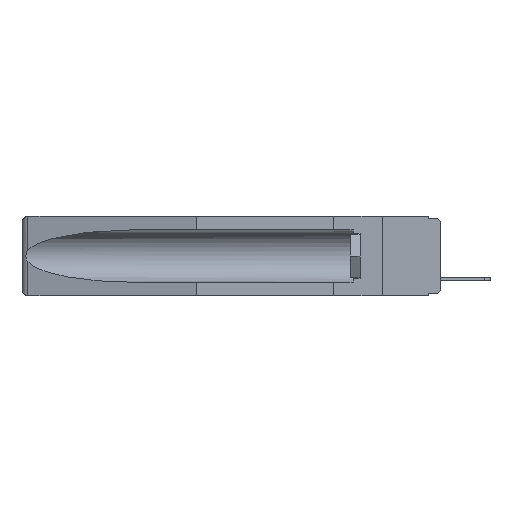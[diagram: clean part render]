
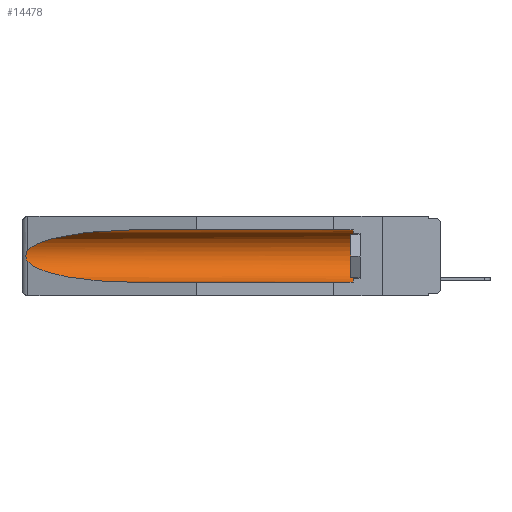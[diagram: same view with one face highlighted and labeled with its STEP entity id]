
A CAD part, left-side view. The second image highlights one B-rep face of the part: STEP entity #14478.
In plain terms, the highlighted cylindrical face has radius 2.857 mm (diameter 5.715 mm), a partial arc.
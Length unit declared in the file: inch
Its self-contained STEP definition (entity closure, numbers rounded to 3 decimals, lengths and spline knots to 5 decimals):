
#69 = CARTESIAN_POINT ( 'NONE',  ( 0.21114, 1.30732, -0.284 ) ) ;
#1136 = CARTESIAN_POINT ( 'NONE',  ( 0.2675, 1.53308, -0.17534 ) ) ;
#1635 = CIRCLE ( 'NONE', #4038, 0.1125 ) ;
#2344 = ORIENTED_EDGE ( 'NONE', *, *, #16342, .T. ) ;
#2562 = CARTESIAN_POINT ( 'NONE',  ( 0.2673, 1.5327, -0.16383 ) ) ;
#2883 = VERTEX_POINT ( 'NONE', #8727 ) ;
#2913 = CARTESIAN_POINT ( 'NONE',  ( 0.155, 1.07973, -0.059 ) ) ;
#2951 = VERTEX_POINT ( 'NONE', #15266 ) ;
#3969 = CARTESIAN_POINT ( 'NONE',  ( 0.26537, 1.52718, -0.14972 ) ) ;
#4036 = DIRECTION ( 'NONE',  ( 0., 1., 0. ) ) ;
#4038 = AXIS2_PLACEMENT_3D ( 'NONE', #18597, #11522, #12834 ) ;
#4839 = EDGE_CURVE ( 'NONE', #2883, #8540, #10561, .T. ) ;
#5042 = CARTESIAN_POINT ( 'NONE',  ( 0.155, -0.30754, -0.1715 ) ) ;
#5213 = VERTEX_POINT ( 'NONE', #5336 ) ;
#5292 = CARTESIAN_POINT ( 'NONE',  ( 0.155, 1.07973, -0.284 ) ) ;
#5336 = CARTESIAN_POINT ( 'NONE',  ( 0.155, 0.126, -0.059 ) ) ;
#5337 = ORIENTED_EDGE ( 'NONE', *, *, #6023, .T. ) ;
#5570 = CARTESIAN_POINT ( 'NONE',  ( 0.26537, 1.52718, -0.19328 ) ) ;
#6023 = EDGE_CURVE ( 'NONE', #2951, #2883, #7710, .T. ) ;
#6224 = CARTESIAN_POINT ( 'NONE',  ( 0.26537, 1.52718, -0.14972 ) ) ;
#6354 = CYLINDRICAL_SURFACE ( 'NONE', #13358, 0.1125 ) ;
#6381 = LINE ( 'NONE', #10812, #17502 ) ;
#6879 = CARTESIAN_POINT ( 'NONE',  ( 0.2673, 1.53269, -0.17917 ) ) ;
#6930 = VECTOR ( 'NONE', #17506, 39.37008 ) ;
#7071 = ORIENTED_EDGE ( 'NONE', *, *, #10542, .T. ) ;
#7710 = B_SPLINE_CURVE_WITH_KNOTS ( 'NONE', 3,
 ( #3969, #9711, #15445, #2562, #14037, #1136, #6879, #10001, #13103, #5570 ),
 .UNSPECIFIED., .F., .F.,
 ( 4, 2, 2, 2, 4 ),
 ( 0., 0.00029, 0.00058, 0.00087, 0.00117 ),
 .UNSPECIFIED. ) ;
#8540 = VERTEX_POINT ( 'NONE', #17273 ) ;
#8727 = CARTESIAN_POINT ( 'NONE',  ( 0.26537, 1.52718, -0.19328 ) ) ;
#8989 = ORIENTED_EDGE ( 'NONE', *, *, #14604, .T. ) ;
#9711 = CARTESIAN_POINT ( 'NONE',  ( 0.26597, 1.52961, -0.15275 ) ) ;
#10001 = CARTESIAN_POINT ( 'NONE',  ( 0.26655, 1.53094, -0.18657 ) ) ;
#10074 = LINE ( 'NONE', #10352, #6930 ) ;
#10352 = CARTESIAN_POINT ( 'NONE',  ( 0.155, -0.30754, -0.059 ) ) ;
#10542 = EDGE_CURVE ( 'NONE', #5213, #11722, #10074, .T. ) ;
#10550 = CARTESIAN_POINT ( 'NONE',  ( 0.155, 1.07973, -0.059 ) ) ;
#10561 =( BOUNDED_CURVE ( )  B_SPLINE_CURVE ( 3, ( #18097, #16784, #69, #5292 ),
 .UNSPECIFIED., .F., .T. ) 
 B_SPLINE_CURVE_WITH_KNOTS ( ( 4, 4 ),
 ( 0.1948, 1.5708 ),
 .UNSPECIFIED. ) 
 CURVE ( )  GEOMETRIC_REPRESENTATION_ITEM ( )  RATIONAL_B_SPLINE_CURVE ( ( 1., 0.848, 0.848, 1. ) ) 
 REPRESENTATION_ITEM ( '' )  );
#10803 = ORIENTED_EDGE ( 'NONE', *, *, #12006, .F. ) ;
#10812 = CARTESIAN_POINT ( 'NONE',  ( 0.155, -0.30754, -0.284 ) ) ;
#11522 = DIRECTION ( 'NONE',  ( 0., -1., 0. ) ) ;
#11591 = CARTESIAN_POINT ( 'NONE',  ( 0.25451, 1.48313, -0.09465 ) ) ;
#11722 = VERTEX_POINT ( 'NONE', #2913 ) ;
#12006 = EDGE_CURVE ( 'NONE', #12168, #8540, #6381, .T. ) ;
#12168 = VERTEX_POINT ( 'NONE', #17211 ) ;
#12467 = DIRECTION ( 'NONE',  ( 0., 1., 0. ) ) ;
#12834 = DIRECTION ( 'NONE',  ( 0., 0., 1. ) ) ;
#13103 = CARTESIAN_POINT ( 'NONE',  ( 0.26597, 1.5296, -0.19026 ) ) ;
#13358 = AXIS2_PLACEMENT_3D ( 'NONE', #5042, #12467, #17932 ) ;
#13596 =( BOUNDED_CURVE ( )  B_SPLINE_CURVE ( 3, ( #10550, #17705, #11591, #6224 ),
 .UNSPECIFIED., .F., .T. ) 
 B_SPLINE_CURVE_WITH_KNOTS ( ( 4, 4 ),
 ( 4.71239, 6.08839 ),
 .UNSPECIFIED. ) 
 CURVE ( )  GEOMETRIC_REPRESENTATION_ITEM ( )  RATIONAL_B_SPLINE_CURVE ( ( 1., 0.848, 0.848, 1. ) ) 
 REPRESENTATION_ITEM ( '' )  );
#14037 = CARTESIAN_POINT ( 'NONE',  ( 0.2675, 1.53308, -0.16763 ) ) ;
#14478 = ADVANCED_FACE ( 'NONE', ( #18220 ), #6354, .F. ) ;
#14604 = EDGE_CURVE ( 'NONE', #12168, #5213, #1635, .T. ) ;
#14903 = EDGE_LOOP ( 'NONE', ( #2344, #5337, #17126, #10803, #8989, #7071 ) ) ;
#15266 = CARTESIAN_POINT ( 'NONE',  ( 0.26537, 1.52718, -0.14972 ) ) ;
#15445 = CARTESIAN_POINT ( 'NONE',  ( 0.26654, 1.53092, -0.15636 ) ) ;
#16342 = EDGE_CURVE ( 'NONE', #11722, #2951, #13596, .T. ) ;
#16784 = CARTESIAN_POINT ( 'NONE',  ( 0.25451, 1.48313, -0.24835 ) ) ;
#17126 = ORIENTED_EDGE ( 'NONE', *, *, #4839, .T. ) ;
#17211 = CARTESIAN_POINT ( 'NONE',  ( 0.155, 0.126, -0.284 ) ) ;
#17273 = CARTESIAN_POINT ( 'NONE',  ( 0.155, 1.07973, -0.284 ) ) ;
#17502 = VECTOR ( 'NONE', #4036, 39.37008 ) ;
#17506 = DIRECTION ( 'NONE',  ( 0., 1., 0. ) ) ;
#17705 = CARTESIAN_POINT ( 'NONE',  ( 0.21114, 1.30732, -0.059 ) ) ;
#17932 = DIRECTION ( 'NONE',  ( 0., 0., 1. ) ) ;
#18097 = CARTESIAN_POINT ( 'NONE',  ( 0.26537, 1.52718, -0.19328 ) ) ;
#18220 = FACE_OUTER_BOUND ( 'NONE', #14903, .T. ) ;
#18597 = CARTESIAN_POINT ( 'NONE',  ( 0.155, 0.126, -0.1715 ) ) ;
